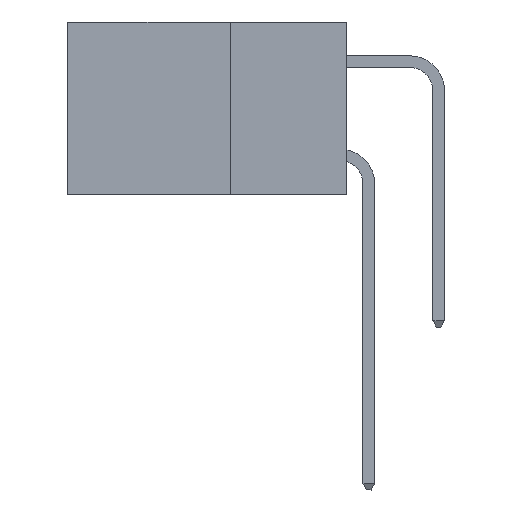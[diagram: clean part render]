
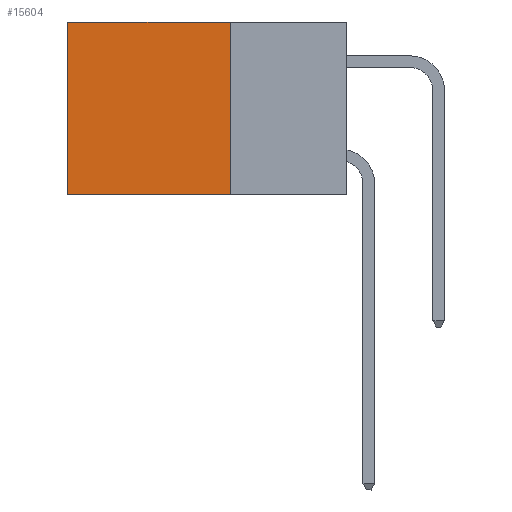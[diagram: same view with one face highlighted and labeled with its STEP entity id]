
A CAD part, left-side view. The second image highlights one B-rep face of the part: STEP entity #15604.
In plain terms, the highlighted planar face has unit normal (-1, 0, 0).
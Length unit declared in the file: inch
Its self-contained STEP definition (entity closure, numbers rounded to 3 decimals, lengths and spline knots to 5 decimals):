
#379 = CARTESIAN_POINT ( 'NONE',  ( 0.2875, 0.6, -0.37 ) ) ;
#1342 = FACE_OUTER_BOUND ( 'NONE', #16539, .T. ) ;
#2889 = DIRECTION ( 'NONE',  ( 0., 1., 0. ) ) ;
#3079 = CARTESIAN_POINT ( 'NONE',  ( 0.2875, 0.25, -0.37 ) ) ;
#6088 = LINE ( 'NONE', #19158, #18238 ) ;
#7518 = CARTESIAN_POINT ( 'NONE',  ( 0.2875, 0.6, 0. ) ) ;
#10626 = AXIS2_PLACEMENT_3D ( 'NONE', #38099, #18670, #11194 ) ;
#11194 = DIRECTION ( 'NONE',  ( 0., 0., -1. ) ) ;
#11221 = CARTESIAN_POINT ( 'NONE',  ( 0.2875, 0.6, 0. ) ) ;
#12714 = LINE ( 'NONE', #3079, #19254 ) ;
#13727 = VECTOR ( 'NONE', #32270, 39.37008 ) ;
#14215 = LINE ( 'NONE', #11221, #36273 ) ;
#15604 = ADVANCED_FACE ( 'NONE', ( #1342 ), #37675, .F. ) ;
#16539 = EDGE_LOOP ( 'NONE', ( #39011, #26662, #27001, #27544 ) ) ;
#18238 = VECTOR ( 'NONE', #2889, 39.37008 ) ;
#18670 = DIRECTION ( 'NONE',  ( 1., 0., 0. ) ) ;
#19158 = CARTESIAN_POINT ( 'NONE',  ( 0.2875, 0.25, 0. ) ) ;
#19254 = VECTOR ( 'NONE', #22760, 39.37008 ) ;
#22422 = VERTEX_POINT ( 'NONE', #22694 ) ;
#22694 = CARTESIAN_POINT ( 'NONE',  ( 0.2875, 0.25, -0.37 ) ) ;
#22760 = DIRECTION ( 'NONE',  ( 0., 1., 0. ) ) ;
#23874 = VERTEX_POINT ( 'NONE', #379 ) ;
#24455 = DIRECTION ( 'NONE',  ( 0., 0., -1. ) ) ;
#26489 = CARTESIAN_POINT ( 'NONE',  ( 0.2875, 0.25, 0. ) ) ;
#26662 = ORIENTED_EDGE ( 'NONE', *, *, #36884, .F. ) ;
#27001 = ORIENTED_EDGE ( 'NONE', *, *, #34565, .F. ) ;
#27544 = ORIENTED_EDGE ( 'NONE', *, *, #28918, .T. ) ;
#28341 = VERTEX_POINT ( 'NONE', #7518 ) ;
#28918 = EDGE_CURVE ( 'NONE', #33661, #28341, #6088, .T. ) ;
#30006 = CARTESIAN_POINT ( 'NONE',  ( 0.2875, 0.25, 0. ) ) ;
#32270 = DIRECTION ( 'NONE',  ( 0., 0., -1. ) ) ;
#33661 = VERTEX_POINT ( 'NONE', #30006 ) ;
#34565 = EDGE_CURVE ( 'NONE', #33661, #22422, #39111, .T. ) ;
#35229 = EDGE_CURVE ( 'NONE', #28341, #23874, #14215, .T. ) ;
#36273 = VECTOR ( 'NONE', #24455, 39.37008 ) ;
#36884 = EDGE_CURVE ( 'NONE', #22422, #23874, #12714, .T. ) ;
#37675 = PLANE ( 'NONE',  #10626 ) ;
#38099 = CARTESIAN_POINT ( 'NONE',  ( 0.2875, 0.25, 0. ) ) ;
#39011 = ORIENTED_EDGE ( 'NONE', *, *, #35229, .T. ) ;
#39111 = LINE ( 'NONE', #26489, #13727 ) ;
